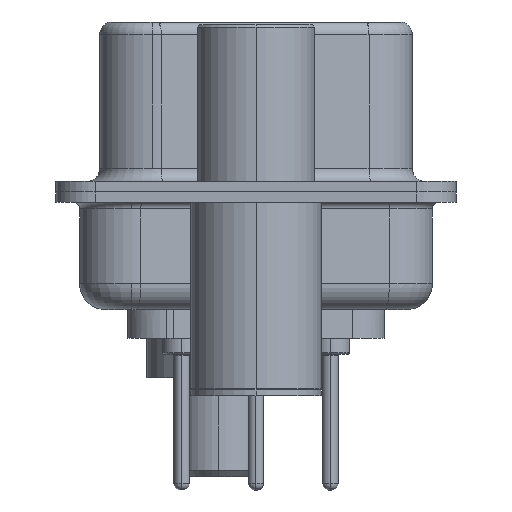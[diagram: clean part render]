
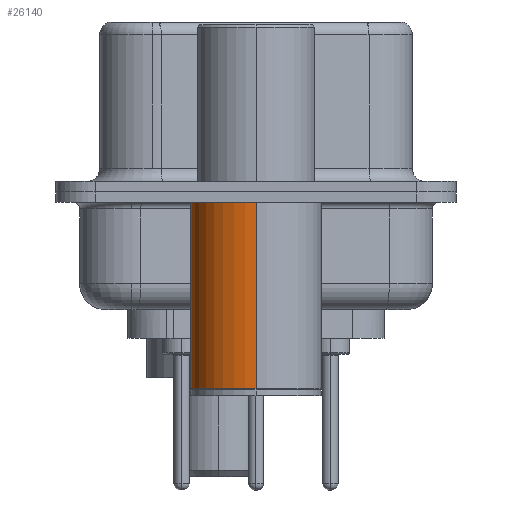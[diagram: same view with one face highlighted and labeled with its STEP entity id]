
A CAD part, left-side view. The second image highlights one B-rep face of the part: STEP entity #26140.
In plain terms, the highlighted cylindrical face has radius 2.5 mm (diameter 5 mm), a partial arc.
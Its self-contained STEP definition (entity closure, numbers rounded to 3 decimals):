
#773 = VECTOR ( 'NONE', #18377, 1000. ) ;
#1970 = DIRECTION ( 'NONE',  ( 1., 0., 0. ) ) ;
#2419 = CIRCLE ( 'NONE', #8679, 2.5 ) ;
#4095 = CYLINDRICAL_SURFACE ( 'NONE', #25782, 2.5 ) ;
#4307 = DIRECTION ( 'NONE',  ( 0., 0., 1. ) ) ;
#5722 = EDGE_CURVE ( 'NONE', #6833, #21557, #28821, .T. ) ;
#6784 = DIRECTION ( 'NONE',  ( 0., 0., 1. ) ) ;
#6833 = VERTEX_POINT ( 'NONE', #16766 ) ;
#8004 = DIRECTION ( 'NONE',  ( 1., 0., 0. ) ) ;
#8180 = VECTOR ( 'NONE', #6784, 1000. ) ;
#8532 = EDGE_CURVE ( 'NONE', #21557, #9015, #15419, .T. ) ;
#8679 = AXIS2_PLACEMENT_3D ( 'NONE', #29107, #12711, #31883 ) ;
#9015 = VERTEX_POINT ( 'NONE', #33494 ) ;
#10441 = ORIENTED_EDGE ( 'NONE', *, *, #5722, .T. ) ;
#12711 = DIRECTION ( 'NONE',  ( 0., 0., 1. ) ) ;
#12855 = EDGE_CURVE ( 'NONE', #29528, #9015, #2419, .T. ) ;
#12917 = DIRECTION ( 'NONE',  ( 0., 0., 1. ) ) ;
#13257 = CARTESIAN_POINT ( 'NONE',  ( 2.5, 0., -0.4 ) ) ;
#13799 = EDGE_LOOP ( 'NONE', ( #10441, #22707, #32153, #21765 ) ) ;
#13815 = CARTESIAN_POINT ( 'NONE',  ( -2.5, 0., -7.525 ) ) ;
#15252 = LINE ( 'NONE', #34789, #773 ) ;
#15419 = LINE ( 'NONE', #18255, #8180 ) ;
#15643 = CARTESIAN_POINT ( 'NONE',  ( 0., 0., 0.581 ) ) ;
#16683 = CARTESIAN_POINT ( 'NONE',  ( 0., 0., -7.525 ) ) ;
#16766 = CARTESIAN_POINT ( 'NONE',  ( 2.5, 0., -7.525 ) ) ;
#18255 = CARTESIAN_POINT ( 'NONE',  ( -2.5, 0., 0.581 ) ) ;
#18377 = DIRECTION ( 'NONE',  ( 0., 0., 1. ) ) ;
#21557 = VERTEX_POINT ( 'NONE', #13815 ) ;
#21765 = ORIENTED_EDGE ( 'NONE', *, *, #22012, .F. ) ;
#22012 = EDGE_CURVE ( 'NONE', #6833, #29528, #15252, .T. ) ;
#22707 = ORIENTED_EDGE ( 'NONE', *, *, #8532, .T. ) ;
#25782 = AXIS2_PLACEMENT_3D ( 'NONE', #15643, #12917, #1970 ) ;
#26140 = ADVANCED_FACE ( 'NONE', ( #34080 ), #4095, .T. ) ;
#26871 = AXIS2_PLACEMENT_3D ( 'NONE', #16683, #4307, #8004 ) ;
#28821 = CIRCLE ( 'NONE', #26871, 2.5 ) ;
#29107 = CARTESIAN_POINT ( 'NONE',  ( 0., 0., -0.4 ) ) ;
#29528 = VERTEX_POINT ( 'NONE', #13257 ) ;
#31883 = DIRECTION ( 'NONE',  ( 1., 0., 0. ) ) ;
#32153 = ORIENTED_EDGE ( 'NONE', *, *, #12855, .F. ) ;
#33494 = CARTESIAN_POINT ( 'NONE',  ( -2.5, 0., -0.4 ) ) ;
#34080 = FACE_OUTER_BOUND ( 'NONE', #13799, .T. ) ;
#34789 = CARTESIAN_POINT ( 'NONE',  ( 2.5, 0., 0.581 ) ) ;
